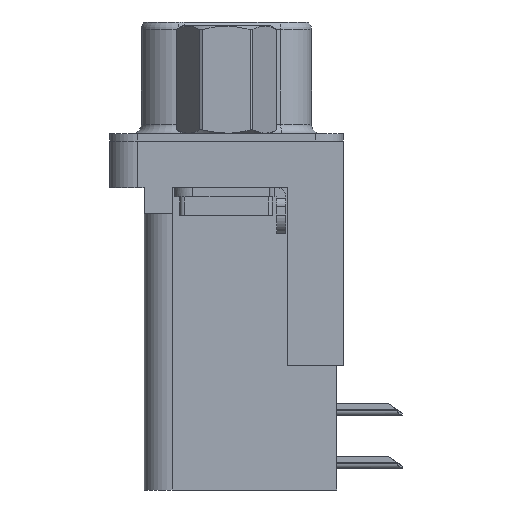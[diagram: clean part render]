
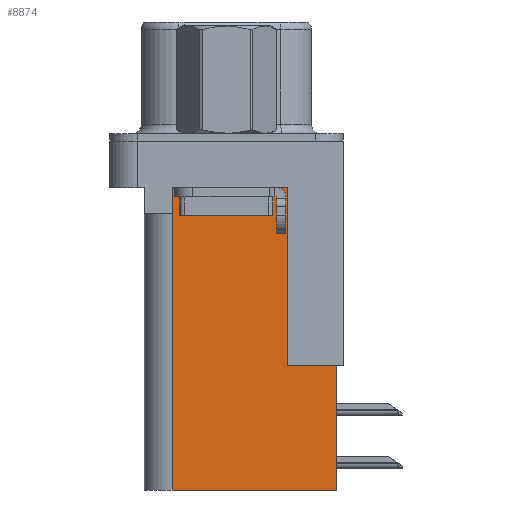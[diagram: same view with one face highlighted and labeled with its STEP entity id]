
A CAD part, left-side view. The second image highlights one B-rep face of the part: STEP entity #8874.
In plain terms, the highlighted planar face has unit normal (-1, 0, 0).
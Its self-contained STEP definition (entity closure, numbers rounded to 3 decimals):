
#399 = EDGE_CURVE ( 'NONE', #16446, #27140, #18793, .T. ) ;
#454 = CARTESIAN_POINT ( 'NONE',  ( 3.7, 2.895, -3.9 ) ) ;
#830 = CARTESIAN_POINT ( 'NONE',  ( 3.7, -3.295, -2.5 ) ) ;
#1183 = LINE ( 'NONE', #23149, #12364 ) ;
#2305 = LINE ( 'NONE', #20356, #7847 ) ;
#2320 = ORIENTED_EDGE ( 'NONE', *, *, #21723, .F. ) ;
#2353 = AXIS2_PLACEMENT_3D ( 'NONE', #5112, #20048, #7205 ) ;
#2848 = EDGE_CURVE ( 'NONE', #17014, #16656, #1183, .T. ) ;
#3639 = FACE_OUTER_BOUND ( 'NONE', #7739, .T. ) ;
#4202 = VECTOR ( 'NONE', #21138, 1000. ) ;
#4709 = LINE ( 'NONE', #11610, #26083 ) ;
#5112 = CARTESIAN_POINT ( 'NONE',  ( 3.7, -3.295, -18.76 ) ) ;
#5441 = VERTEX_POINT ( 'NONE', #22879 ) ;
#5483 = ORIENTED_EDGE ( 'NONE', *, *, #8950, .F. ) ;
#5862 = ORIENTED_EDGE ( 'NONE', *, *, #10918, .T. ) ;
#5939 = CARTESIAN_POINT ( 'NONE',  ( 3.7, -5.925, -12.05 ) ) ;
#7205 = DIRECTION ( 'NONE',  ( 0., 1., 0. ) ) ;
#7310 = EDGE_CURVE ( 'NONE', #5441, #17014, #18279, .T. ) ;
#7711 = EDGE_CURVE ( 'NONE', #9336, #25292, #9234, .T. ) ;
#7739 = EDGE_LOOP ( 'NONE', ( #11841, #5862, #15072, #5483, #26145, #2320, #19867, #21866 ) ) ;
#7847 = VECTOR ( 'NONE', #22373, 1000. ) ;
#8119 = VECTOR ( 'NONE', #12841, 1000. ) ;
#8502 = CARTESIAN_POINT ( 'NONE',  ( 3.7, -6.295, -12.05 ) ) ;
#8874 = ADVANCED_FACE ( 'NONE', ( #3639 ), #17883, .F. ) ;
#8950 = EDGE_CURVE ( 'NONE', #27140, #25292, #2305, .T. ) ;
#9234 = LINE ( 'NONE', #12423, #19285 ) ;
#9336 = VERTEX_POINT ( 'NONE', #454 ) ;
#9882 = VECTOR ( 'NONE', #12345, 1000. ) ;
#10807 = VERTEX_POINT ( 'NONE', #5939 ) ;
#10918 = EDGE_CURVE ( 'NONE', #16656, #9336, #15814, .T. ) ;
#11610 = CARTESIAN_POINT ( 'NONE',  ( 3.7, -5.925, -2. ) ) ;
#11841 = ORIENTED_EDGE ( 'NONE', *, *, #2848, .T. ) ;
#12345 = DIRECTION ( 'NONE',  ( 0., 0., 1. ) ) ;
#12364 = VECTOR ( 'NONE', #22501, 1000. ) ;
#12423 = CARTESIAN_POINT ( 'NONE',  ( 3.7, 0., -3.9 ) ) ;
#12604 = CARTESIAN_POINT ( 'NONE',  ( 3.7, 2.925, -3.9 ) ) ;
#12841 = DIRECTION ( 'NONE',  ( 0., 1., 0. ) ) ;
#13791 = DIRECTION ( 'NONE',  ( 0., 0., -1. ) ) ;
#13796 = VECTOR ( 'NONE', #18235, 1000. ) ;
#13848 = LINE ( 'NONE', #8502, #8119 ) ;
#15072 = ORIENTED_EDGE ( 'NONE', *, *, #7711, .T. ) ;
#15814 = LINE ( 'NONE', #18953, #4202 ) ;
#16446 = VERTEX_POINT ( 'NONE', #24237 ) ;
#16656 = VERTEX_POINT ( 'NONE', #24689 ) ;
#17014 = VERTEX_POINT ( 'NONE', #830 ) ;
#17883 = PLANE ( 'NONE',  #2353 ) ;
#18235 = DIRECTION ( 'NONE',  ( 0., 1., 0. ) ) ;
#18279 = LINE ( 'NONE', #18707, #9882 ) ;
#18707 = CARTESIAN_POINT ( 'NONE',  ( 3.7, -3.295, -18.76 ) ) ;
#18778 = DIRECTION ( 'NONE',  ( 0., 1., 0. ) ) ;
#18793 = LINE ( 'NONE', #22916, #13796 ) ;
#18953 = CARTESIAN_POINT ( 'NONE',  ( 3.7, 2.895, -3.9 ) ) ;
#19285 = VECTOR ( 'NONE', #18778, 1000. ) ;
#19309 = EDGE_CURVE ( 'NONE', #10807, #5441, #13848, .T. ) ;
#19867 = ORIENTED_EDGE ( 'NONE', *, *, #19309, .T. ) ;
#20048 = DIRECTION ( 'NONE',  ( 1., 0., 0. ) ) ;
#20356 = CARTESIAN_POINT ( 'NONE',  ( 3.7, 2.925, -18.76 ) ) ;
#21138 = DIRECTION ( 'NONE',  ( 0., 0., -1. ) ) ;
#21723 = EDGE_CURVE ( 'NONE', #10807, #16446, #4709, .T. ) ;
#21866 = ORIENTED_EDGE ( 'NONE', *, *, #7310, .T. ) ;
#22373 = DIRECTION ( 'NONE',  ( 0., 0., 1. ) ) ;
#22501 = DIRECTION ( 'NONE',  ( 0., 1., 0. ) ) ;
#22879 = CARTESIAN_POINT ( 'NONE',  ( 3.7, -3.295, -12.05 ) ) ;
#22916 = CARTESIAN_POINT ( 'NONE',  ( 3.7, -3.295, -18.76 ) ) ;
#23149 = CARTESIAN_POINT ( 'NONE',  ( 3.7, -3.295, -2.5 ) ) ;
#24237 = CARTESIAN_POINT ( 'NONE',  ( 3.7, -5.925, -18.76 ) ) ;
#24689 = CARTESIAN_POINT ( 'NONE',  ( 3.7, 2.895, -2.5 ) ) ;
#25089 = CARTESIAN_POINT ( 'NONE',  ( 3.7, 2.925, -18.76 ) ) ;
#25292 = VERTEX_POINT ( 'NONE', #12604 ) ;
#26083 = VECTOR ( 'NONE', #13791, 1000. ) ;
#26145 = ORIENTED_EDGE ( 'NONE', *, *, #399, .F. ) ;
#27140 = VERTEX_POINT ( 'NONE', #25089 ) ;
